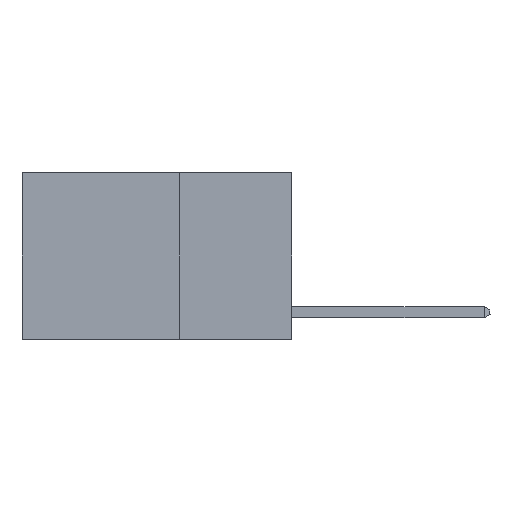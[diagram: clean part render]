
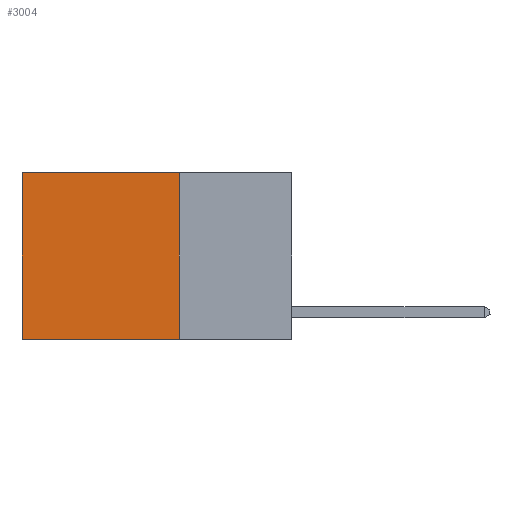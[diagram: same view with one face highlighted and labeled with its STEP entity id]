
A CAD part, left-side view. The second image highlights one B-rep face of the part: STEP entity #3004.
In plain terms, the highlighted planar face has unit normal (-1, 0, 0).
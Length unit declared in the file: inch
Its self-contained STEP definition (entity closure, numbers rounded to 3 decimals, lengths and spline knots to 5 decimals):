
#69 = CARTESIAN_POINT ( 'NONE',  ( 0.2625, 0.25, -0.37 ) ) ;
#183 = ORIENTED_EDGE ( 'NONE', *, *, #3033, .F. ) ;
#215 = PLANE ( 'NONE',  #8847 ) ;
#951 = EDGE_CURVE ( 'NONE', #8575, #5600, #6981, .T. ) ;
#1126 = EDGE_LOOP ( 'NONE', ( #8292, #183, #2457, #4589 ) ) ;
#1157 = DIRECTION ( 'NONE',  ( 1., 0., 0. ) ) ;
#1238 = CARTESIAN_POINT ( 'NONE',  ( 0.2625, 0.25, 0. ) ) ;
#1578 = CARTESIAN_POINT ( 'NONE',  ( 0.2625, 0.25, 0. ) ) ;
#1580 = CARTESIAN_POINT ( 'NONE',  ( 0.2625, 0.25, 0. ) ) ;
#2457 = ORIENTED_EDGE ( 'NONE', *, *, #2717, .F. ) ;
#2717 = EDGE_CURVE ( 'NONE', #8575, #9303, #6250, .T. ) ;
#3004 = ADVANCED_FACE ( 'NONE', ( #9365 ), #215, .F. ) ;
#3033 = EDGE_CURVE ( 'NONE', #9303, #3808, #3365, .T. ) ;
#3257 = VECTOR ( 'NONE', #9934, 39.37008 ) ;
#3365 = LINE ( 'NONE', #5935, #5203 ) ;
#3582 = CARTESIAN_POINT ( 'NONE',  ( 0.2625, 0.25, 0. ) ) ;
#3808 = VERTEX_POINT ( 'NONE', #3982 ) ;
#3982 = CARTESIAN_POINT ( 'NONE',  ( 0.2625, 0.6, -0.37 ) ) ;
#4244 = VECTOR ( 'NONE', #7007, 39.37008 ) ;
#4589 = ORIENTED_EDGE ( 'NONE', *, *, #951, .T. ) ;
#4770 = VECTOR ( 'NONE', #7287, 39.37008 ) ;
#5203 = VECTOR ( 'NONE', #8155, 39.37008 ) ;
#5600 = VERTEX_POINT ( 'NONE', #5723 ) ;
#5723 = CARTESIAN_POINT ( 'NONE',  ( 0.2625, 0.6, 0. ) ) ;
#5935 = CARTESIAN_POINT ( 'NONE',  ( 0.2625, 0.25, -0.37 ) ) ;
#6250 = LINE ( 'NONE', #1580, #4244 ) ;
#6649 = DIRECTION ( 'NONE',  ( 0., 0., -1. ) ) ;
#6981 = LINE ( 'NONE', #1578, #4770 ) ;
#7007 = DIRECTION ( 'NONE',  ( 0., 0., -1. ) ) ;
#7287 = DIRECTION ( 'NONE',  ( 0., 1., 0. ) ) ;
#8155 = DIRECTION ( 'NONE',  ( 0., 1., 0. ) ) ;
#8292 = ORIENTED_EDGE ( 'NONE', *, *, #9000, .T. ) ;
#8439 = CARTESIAN_POINT ( 'NONE',  ( 0.2625, 0.6, 0. ) ) ;
#8575 = VERTEX_POINT ( 'NONE', #1238 ) ;
#8847 = AXIS2_PLACEMENT_3D ( 'NONE', #3582, #1157, #6649 ) ;
#9000 = EDGE_CURVE ( 'NONE', #5600, #3808, #9259, .T. ) ;
#9259 = LINE ( 'NONE', #8439, #3257 ) ;
#9303 = VERTEX_POINT ( 'NONE', #69 ) ;
#9365 = FACE_OUTER_BOUND ( 'NONE', #1126, .T. ) ;
#9934 = DIRECTION ( 'NONE',  ( 0., 0., -1. ) ) ;
